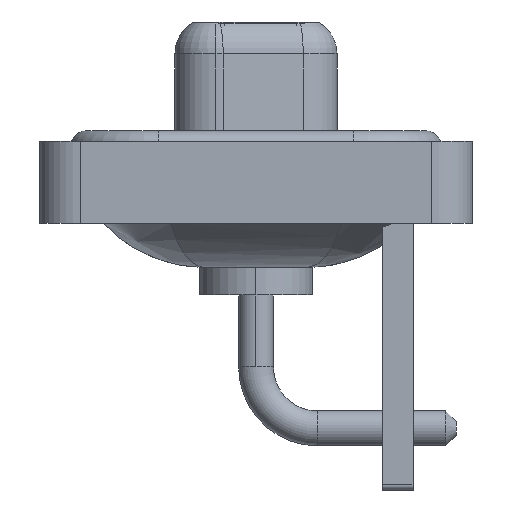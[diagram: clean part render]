
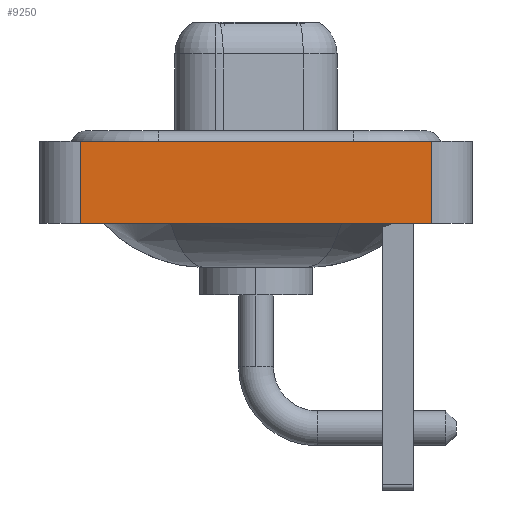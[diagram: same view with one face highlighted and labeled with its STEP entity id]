
A CAD part, left-side view. The second image highlights one B-rep face of the part: STEP entity #9250.
In plain terms, the highlighted planar face has unit normal (-1, 0, 0).
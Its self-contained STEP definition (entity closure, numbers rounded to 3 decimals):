
#353 = CARTESIAN_POINT ( 'NONE',  ( -7.3, -8.55, -3.6 ) ) ;
#529 = DIRECTION ( 'NONE',  ( 0., 0., 1. ) ) ;
#1411 = EDGE_CURVE ( 'NONE', #12510, #2204, #1793, .T. ) ;
#1683 = DIRECTION ( 'NONE',  ( 0., 0., 1. ) ) ;
#1752 = VERTEX_POINT ( 'NONE', #10941 ) ;
#1793 = LINE ( 'NONE', #6973, #10773 ) ;
#1956 = PLANE ( 'NONE',  #5003 ) ;
#2204 = VERTEX_POINT ( 'NONE', #15525 ) ;
#2398 = ORIENTED_EDGE ( 'NONE', *, *, #10031, .T. ) ;
#3019 = CARTESIAN_POINT ( 'NONE',  ( -7.3, -8.55, 0.4 ) ) ;
#3487 = EDGE_CURVE ( 'NONE', #1752, #11244, #9238, .T. ) ;
#4078 = DIRECTION ( 'NONE',  ( 0., -1., 0. ) ) ;
#4439 = VECTOR ( 'NONE', #1683, 1000. ) ;
#4492 = FACE_OUTER_BOUND ( 'NONE', #8596, .T. ) ;
#5003 = AXIS2_PLACEMENT_3D ( 'NONE', #353, #5615, #529 ) ;
#5615 = DIRECTION ( 'NONE',  ( -1., 0., 0. ) ) ;
#6840 = CARTESIAN_POINT ( 'NONE',  ( -7.3, -8.55, -3.6 ) ) ;
#6973 = CARTESIAN_POINT ( 'NONE',  ( -7.3, -8.55, -3.6 ) ) ;
#8212 = CARTESIAN_POINT ( 'NONE',  ( -7.3, 8.55, -3.6 ) ) ;
#8596 = EDGE_LOOP ( 'NONE', ( #2398, #14380, #10845, #9141 ) ) ;
#9141 = ORIENTED_EDGE ( 'NONE', *, *, #1411, .T. ) ;
#9238 = LINE ( 'NONE', #3019, #12749 ) ;
#9250 = ADVANCED_FACE ( 'NONE', ( #4492 ), #1956, .T. ) ;
#9666 = LINE ( 'NONE', #16136, #4439 ) ;
#10031 = EDGE_CURVE ( 'NONE', #2204, #11244, #10684, .T. ) ;
#10499 = VECTOR ( 'NONE', #13413, 1000. ) ;
#10684 = LINE ( 'NONE', #6840, #10499 ) ;
#10773 = VECTOR ( 'NONE', #4078, 1000. ) ;
#10845 = ORIENTED_EDGE ( 'NONE', *, *, #16553, .F. ) ;
#10941 = CARTESIAN_POINT ( 'NONE',  ( -7.3, 8.55, 0.4 ) ) ;
#11244 = VERTEX_POINT ( 'NONE', #11374 ) ;
#11374 = CARTESIAN_POINT ( 'NONE',  ( -7.3, -8.55, 0.4 ) ) ;
#12510 = VERTEX_POINT ( 'NONE', #8212 ) ;
#12749 = VECTOR ( 'NONE', #15965, 1000. ) ;
#13413 = DIRECTION ( 'NONE',  ( 0., 0., 1. ) ) ;
#14380 = ORIENTED_EDGE ( 'NONE', *, *, #3487, .F. ) ;
#15525 = CARTESIAN_POINT ( 'NONE',  ( -7.3, -8.55, -3.6 ) ) ;
#15965 = DIRECTION ( 'NONE',  ( 0., -1., 0. ) ) ;
#16136 = CARTESIAN_POINT ( 'NONE',  ( -7.3, 8.55, -3.6 ) ) ;
#16553 = EDGE_CURVE ( 'NONE', #12510, #1752, #9666, .T. ) ;
